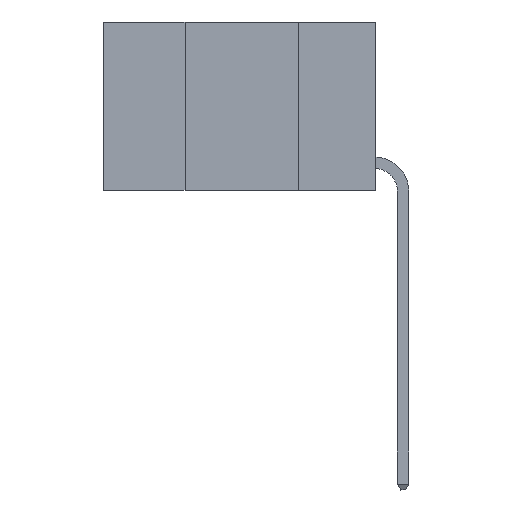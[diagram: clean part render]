
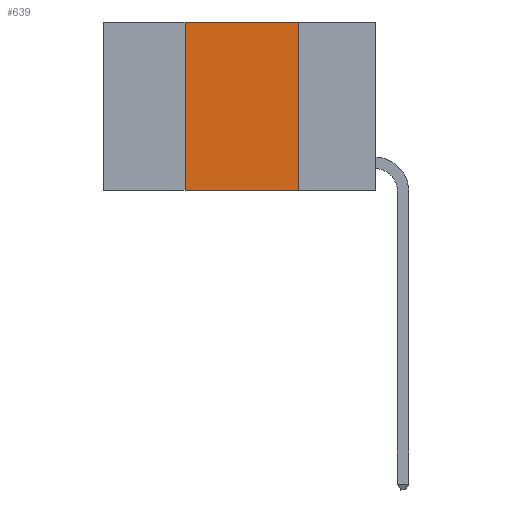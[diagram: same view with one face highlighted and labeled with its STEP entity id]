
A CAD part, left-side view. The second image highlights one B-rep face of the part: STEP entity #639.
In plain terms, the highlighted planar face has unit normal (-1, 0, 0).
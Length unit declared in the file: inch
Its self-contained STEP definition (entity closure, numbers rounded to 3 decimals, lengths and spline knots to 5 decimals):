
#87 = DIRECTION ( 'NONE',  ( 0., 0., -1. ) ) ;
#579 = CARTESIAN_POINT ( 'NONE',  ( 0., 0.42, -0.37 ) ) ;
#594 = ORIENTED_EDGE ( 'NONE', *, *, #5625, .F. ) ;
#639 = ADVANCED_FACE ( 'NONE', ( #4900 ), #5626, .F. ) ;
#978 = DIRECTION ( 'NONE',  ( 0., 0., -1. ) ) ;
#1049 = CARTESIAN_POINT ( 'NONE',  ( 0., 0.42, 0. ) ) ;
#1063 = VECTOR ( 'NONE', #4262, 39.37008 ) ;
#2125 = VERTEX_POINT ( 'NONE', #8422 ) ;
#2299 = LINE ( 'NONE', #8489, #4942 ) ;
#2342 = DIRECTION ( 'NONE',  ( 1., 0., 0. ) ) ;
#3066 = EDGE_LOOP ( 'NONE', ( #594, #7809, #8400, #8219 ) ) ;
#3119 = CARTESIAN_POINT ( 'NONE',  ( 0., 0.6, 0. ) ) ;
#3132 = VERTEX_POINT ( 'NONE', #579 ) ;
#3743 = CARTESIAN_POINT ( 'NONE',  ( 0., 0.17, -0.37 ) ) ;
#3867 = DIRECTION ( 'NONE',  ( 0., -1., 0. ) ) ;
#3961 = EDGE_CURVE ( 'NONE', #3132, #9605, #5836, .T. ) ;
#4262 = DIRECTION ( 'NONE',  ( 0., -1., 0. ) ) ;
#4648 = CARTESIAN_POINT ( 'NONE',  ( 0., 0.6, 0. ) ) ;
#4900 = FACE_OUTER_BOUND ( 'NONE', #3066, .T. ) ;
#4942 = VECTOR ( 'NONE', #6848, 39.37008 ) ;
#5625 = EDGE_CURVE ( 'NONE', #2125, #9605, #7158, .T. ) ;
#5626 = PLANE ( 'NONE',  #9134 ) ;
#5836 = LINE ( 'NONE', #6597, #1063 ) ;
#6597 = CARTESIAN_POINT ( 'NONE',  ( 0., 0.6, -0.37 ) ) ;
#6848 = DIRECTION ( 'NONE',  ( 0., 0., 1. ) ) ;
#7158 = LINE ( 'NONE', #9610, #8935 ) ;
#7809 = ORIENTED_EDGE ( 'NONE', *, *, #9095, .F. ) ;
#8166 = VERTEX_POINT ( 'NONE', #1049 ) ;
#8219 = ORIENTED_EDGE ( 'NONE', *, *, #3961, .T. ) ;
#8374 = LINE ( 'NONE', #4648, #8791 ) ;
#8400 = ORIENTED_EDGE ( 'NONE', *, *, #9525, .F. ) ;
#8422 = CARTESIAN_POINT ( 'NONE',  ( 0., 0.17, 0. ) ) ;
#8489 = CARTESIAN_POINT ( 'NONE',  ( 0., 0.42, 0. ) ) ;
#8791 = VECTOR ( 'NONE', #3867, 39.37008 ) ;
#8935 = VECTOR ( 'NONE', #87, 39.37008 ) ;
#9095 = EDGE_CURVE ( 'NONE', #8166, #2125, #8374, .T. ) ;
#9134 = AXIS2_PLACEMENT_3D ( 'NONE', #3119, #2342, #978 ) ;
#9525 = EDGE_CURVE ( 'NONE', #3132, #8166, #2299, .T. ) ;
#9605 = VERTEX_POINT ( 'NONE', #3743 ) ;
#9610 = CARTESIAN_POINT ( 'NONE',  ( 0., 0.17, 0. ) ) ;
